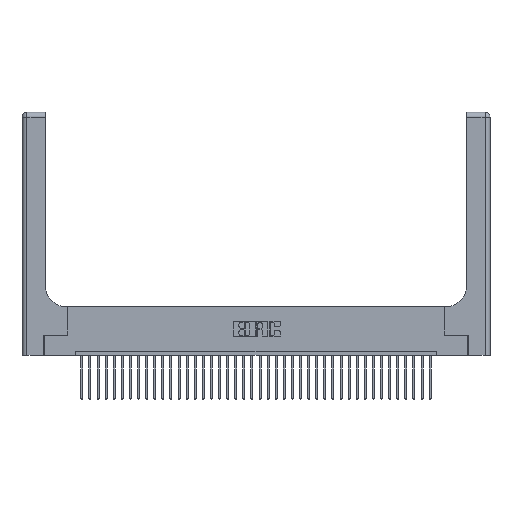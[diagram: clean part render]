
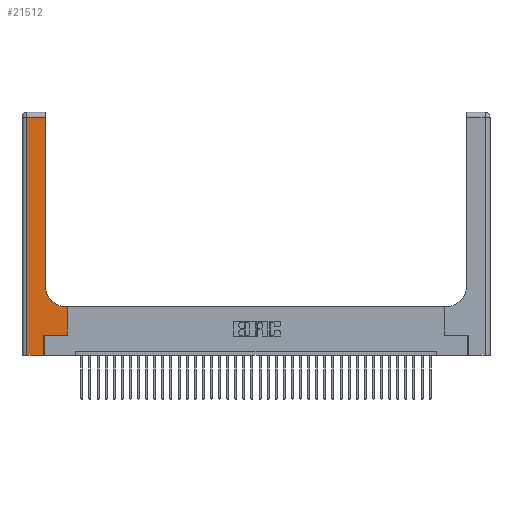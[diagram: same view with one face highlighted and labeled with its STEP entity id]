
A CAD part, top view. The second image highlights one B-rep face of the part: STEP entity #21512.
In plain terms, the highlighted planar face has unit normal (0, 0, 1).
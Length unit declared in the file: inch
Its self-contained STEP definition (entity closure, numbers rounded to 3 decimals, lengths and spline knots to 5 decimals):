
#580 = CARTESIAN_POINT ( 'NONE',  ( 0.269, 0., 0.37 ) ) ;
#659 = DIRECTION ( 'NONE',  ( 1., 0., 0. ) ) ;
#1105 = VECTOR ( 'NONE', #34645, 39.37008 ) ;
#1574 = VECTOR ( 'NONE', #26464, 39.37008 ) ;
#2365 = AXIS2_PLACEMENT_3D ( 'NONE', #33145, #10045, #27324 ) ;
#2456 = LINE ( 'NONE', #13528, #1105 ) ;
#2549 = ORIENTED_EDGE ( 'NONE', *, *, #35047, .T. ) ;
#2622 = ORIENTED_EDGE ( 'NONE', *, *, #21382, .T. ) ;
#2945 = ORIENTED_EDGE ( 'NONE', *, *, #21326, .T. ) ;
#3065 = VERTEX_POINT ( 'NONE', #580 ) ;
#3485 = FACE_OUTER_BOUND ( 'NONE', #27033, .T. ) ;
#4107 = ORIENTED_EDGE ( 'NONE', *, *, #4383, .T. ) ;
#4383 = EDGE_CURVE ( 'NONE', #3065, #17156, #23587, .T. ) ;
#4386 = VECTOR ( 'NONE', #659, 39.37008 ) ;
#4394 = DIRECTION ( 'NONE',  ( 0., -1., 0. ) ) ;
#4868 = EDGE_CURVE ( 'NONE', #8314, #3065, #2456, .T. ) ;
#4983 = ORIENTED_EDGE ( 'NONE', *, *, #15352, .T. ) ;
#5119 = VERTEX_POINT ( 'NONE', #12391 ) ;
#5388 = EDGE_CURVE ( 'NONE', #37314, #37170, #11169, .T. ) ;
#6237 = CARTESIAN_POINT ( 'NONE',  ( 0.5585, 0.25, 0.37 ) ) ;
#7411 = CARTESIAN_POINT ( 'NONE',  ( 0., 2.94, 0.37 ) ) ;
#7849 = CIRCLE ( 'NONE', #29339, 0.25 ) ;
#8225 = CARTESIAN_POINT ( 'NONE',  ( 0.5585, 0.25, 0.37 ) ) ;
#8314 = VERTEX_POINT ( 'NONE', #20662 ) ;
#9167 = CARTESIAN_POINT ( 'NONE',  ( 0.269, 0.25, 0.37 ) ) ;
#10045 = DIRECTION ( 'NONE',  ( 0., 0., -1. ) ) ;
#10732 = DIRECTION ( 'NONE',  ( -1., 0., 0. ) ) ;
#11104 = DIRECTION ( 'NONE',  ( -1., 0., 0. ) ) ;
#11169 = LINE ( 'NONE', #6237, #20300 ) ;
#11295 = ORIENTED_EDGE ( 'NONE', *, *, #23191, .T. ) ;
#11647 = ORIENTED_EDGE ( 'NONE', *, *, #5388, .T. ) ;
#12391 = CARTESIAN_POINT ( 'NONE',  ( 0.2915, 0.85, 0.37 ) ) ;
#13391 = CARTESIAN_POINT ( 'NONE',  ( 0.5585, 0.6, 0.37 ) ) ;
#13528 = CARTESIAN_POINT ( 'NONE',  ( 0., 0., 0.37 ) ) ;
#13589 = VECTOR ( 'NONE', #11104, 39.37008 ) ;
#14628 = VERTEX_POINT ( 'NONE', #18381 ) ;
#14655 = VERTEX_POINT ( 'NONE', #21548 ) ;
#15276 = DIRECTION ( 'NONE',  ( 1., 0., 0. ) ) ;
#15352 = EDGE_CURVE ( 'NONE', #17899, #14628, #23223, .T. ) ;
#15399 = CARTESIAN_POINT ( 'NONE',  ( 0.5415, 0.85, 0.37 ) ) ;
#15915 = VECTOR ( 'NONE', #10732, 39.37008 ) ;
#16040 = EDGE_CURVE ( 'NONE', #37170, #14655, #34688, .T. ) ;
#16343 = CARTESIAN_POINT ( 'NONE',  ( 0.06, 3., 0.37 ) ) ;
#17156 = VERTEX_POINT ( 'NONE', #30898 ) ;
#17899 = VERTEX_POINT ( 'NONE', #28649 ) ;
#18381 = CARTESIAN_POINT ( 'NONE',  ( 0.06, 2.94, 0.37 ) ) ;
#20300 = VECTOR ( 'NONE', #32923, 39.37008 ) ;
#20662 = CARTESIAN_POINT ( 'NONE',  ( 0.06, 0., 0.37 ) ) ;
#20677 = CARTESIAN_POINT ( 'NONE',  ( 0.2915, 3., 0.37 ) ) ;
#20942 = DIRECTION ( 'NONE',  ( 0., 1., 0. ) ) ;
#21213 = LINE ( 'NONE', #16343, #30424 ) ;
#21326 = EDGE_CURVE ( 'NONE', #5119, #17899, #34233, .T. ) ;
#21382 = EDGE_CURVE ( 'NONE', #17156, #37314, #34192, .T. ) ;
#21512 = ADVANCED_FACE ( 'NONE', ( #3485 ), #21704, .F. ) ;
#21548 = CARTESIAN_POINT ( 'NONE',  ( 0.5415, 0.6, 0.37 ) ) ;
#21704 = PLANE ( 'NONE',  #2365 ) ;
#23191 = EDGE_CURVE ( 'NONE', #14628, #8314, #21213, .T. ) ;
#23223 = LINE ( 'NONE', #7411, #15915 ) ;
#23587 = LINE ( 'NONE', #37405, #1574 ) ;
#26464 = DIRECTION ( 'NONE',  ( 0., 1., 0. ) ) ;
#27033 = EDGE_LOOP ( 'NONE', ( #2945, #4983, #11295, #32061, #4107, #2622, #11647, #35490, #2549 ) ) ;
#27147 = DIRECTION ( 'NONE',  ( 0., 0., -1. ) ) ;
#27324 = DIRECTION ( 'NONE',  ( -1., 0., 0. ) ) ;
#28247 = VECTOR ( 'NONE', #20942, 39.37008 ) ;
#28649 = CARTESIAN_POINT ( 'NONE',  ( 0.2915, 2.94, 0.37 ) ) ;
#29339 = AXIS2_PLACEMENT_3D ( 'NONE', #15399, #27147, #15276 ) ;
#30424 = VECTOR ( 'NONE', #4394, 39.37008 ) ;
#30898 = CARTESIAN_POINT ( 'NONE',  ( 0.269, 0.25, 0.37 ) ) ;
#32061 = ORIENTED_EDGE ( 'NONE', *, *, #4868, .T. ) ;
#32923 = DIRECTION ( 'NONE',  ( 0., 1., 0. ) ) ;
#33145 = CARTESIAN_POINT ( 'NONE',  ( 0., 3., 0.37 ) ) ;
#34192 = LINE ( 'NONE', #9167, #4386 ) ;
#34233 = LINE ( 'NONE', #20677, #28247 ) ;
#34645 = DIRECTION ( 'NONE',  ( 1., 0., 0. ) ) ;
#34688 = LINE ( 'NONE', #37358, #13589 ) ;
#35047 = EDGE_CURVE ( 'NONE', #14655, #5119, #7849, .T. ) ;
#35490 = ORIENTED_EDGE ( 'NONE', *, *, #16040, .T. ) ;
#37170 = VERTEX_POINT ( 'NONE', #13391 ) ;
#37314 = VERTEX_POINT ( 'NONE', #8225 ) ;
#37358 = CARTESIAN_POINT ( 'NONE',  ( 0.2915, 0.6, 0.37 ) ) ;
#37405 = CARTESIAN_POINT ( 'NONE',  ( 0.269, 0., 0.37 ) ) ;
